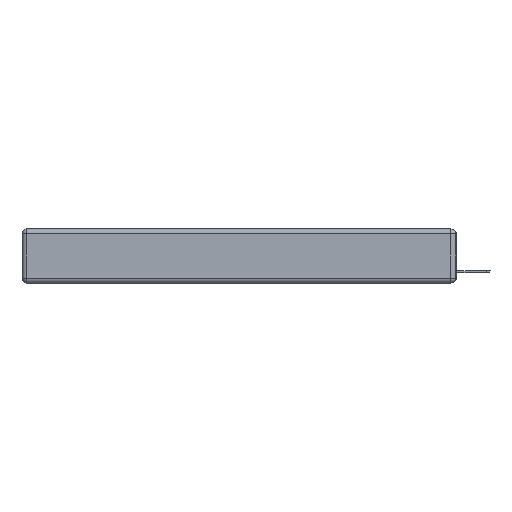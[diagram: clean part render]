
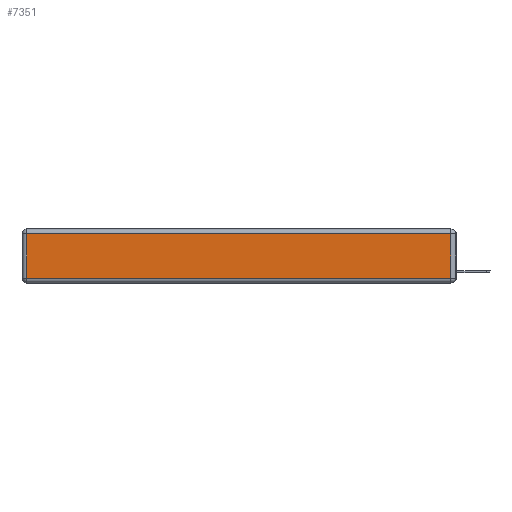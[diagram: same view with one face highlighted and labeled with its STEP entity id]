
A CAD part, left-side view. The second image highlights one B-rep face of the part: STEP entity #7351.
In plain terms, the highlighted planar face has unit normal (-1, 0, 0).
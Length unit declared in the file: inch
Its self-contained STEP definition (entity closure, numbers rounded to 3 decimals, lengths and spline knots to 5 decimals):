
#113 = EDGE_CURVE ( 'NONE', #229, #4045, #10586, .T. ) ;
#229 = VERTEX_POINT ( 'NONE', #14299 ) ;
#1381 = DIRECTION ( 'NONE',  ( 0., 0., 1. ) ) ;
#2094 = LINE ( 'NONE', #6769, #9695 ) ;
#2539 = CARTESIAN_POINT ( 'NONE',  ( 0., 0., -0.343 ) ) ;
#2603 = FACE_OUTER_BOUND ( 'NONE', #2809, .T. ) ;
#2768 = LINE ( 'NONE', #13583, #11820 ) ;
#2809 = EDGE_LOOP ( 'NONE', ( #13010, #4001, #4741, #9688 ) ) ;
#3086 = LINE ( 'NONE', #11426, #7405 ) ;
#4001 = ORIENTED_EDGE ( 'NONE', *, *, #113, .T. ) ;
#4045 = VERTEX_POINT ( 'NONE', #14025 ) ;
#4640 = EDGE_CURVE ( 'NONE', #7079, #229, #3086, .T. ) ;
#4741 = ORIENTED_EDGE ( 'NONE', *, *, #6867, .T. ) ;
#6674 = AXIS2_PLACEMENT_3D ( 'NONE', #2539, #10952, #1381 ) ;
#6769 = CARTESIAN_POINT ( 'NONE',  ( 0., 2.75, -0.03 ) ) ;
#6867 = EDGE_CURVE ( 'NONE', #4045, #14932, #2094, .T. ) ;
#7079 = VERTEX_POINT ( 'NONE', #13892 ) ;
#7351 = ADVANCED_FACE ( 'NONE', ( #2603 ), #14201, .T. ) ;
#7405 = VECTOR ( 'NONE', #14821, 39.37008 ) ;
#8521 = CARTESIAN_POINT ( 'NONE',  ( 0., 2.72, -0.03 ) ) ;
#9688 = ORIENTED_EDGE ( 'NONE', *, *, #12972, .T. ) ;
#9695 = VECTOR ( 'NONE', #11509, 39.37008 ) ;
#10586 = LINE ( 'NONE', #10676, #13005 ) ;
#10676 = CARTESIAN_POINT ( 'NONE',  ( 0., 0.03, -0.343 ) ) ;
#10952 = DIRECTION ( 'NONE',  ( -1., 0., 0. ) ) ;
#11426 = CARTESIAN_POINT ( 'NONE',  ( 0., 0., -0.313 ) ) ;
#11509 = DIRECTION ( 'NONE',  ( 0., 1., 0. ) ) ;
#11820 = VECTOR ( 'NONE', #13667, 39.37008 ) ;
#11908 = DIRECTION ( 'NONE',  ( 0., 0., 1. ) ) ;
#12972 = EDGE_CURVE ( 'NONE', #14932, #7079, #2768, .T. ) ;
#13005 = VECTOR ( 'NONE', #11908, 39.37008 ) ;
#13010 = ORIENTED_EDGE ( 'NONE', *, *, #4640, .T. ) ;
#13583 = CARTESIAN_POINT ( 'NONE',  ( 0., 2.72, -0.343 ) ) ;
#13667 = DIRECTION ( 'NONE',  ( 0., 0., -1. ) ) ;
#13892 = CARTESIAN_POINT ( 'NONE',  ( 0., 2.72, -0.313 ) ) ;
#14025 = CARTESIAN_POINT ( 'NONE',  ( 0., 0.03, -0.03 ) ) ;
#14201 = PLANE ( 'NONE',  #6674 ) ;
#14299 = CARTESIAN_POINT ( 'NONE',  ( 0., 0.03, -0.313 ) ) ;
#14821 = DIRECTION ( 'NONE',  ( 0., -1., 0. ) ) ;
#14932 = VERTEX_POINT ( 'NONE', #8521 ) ;
